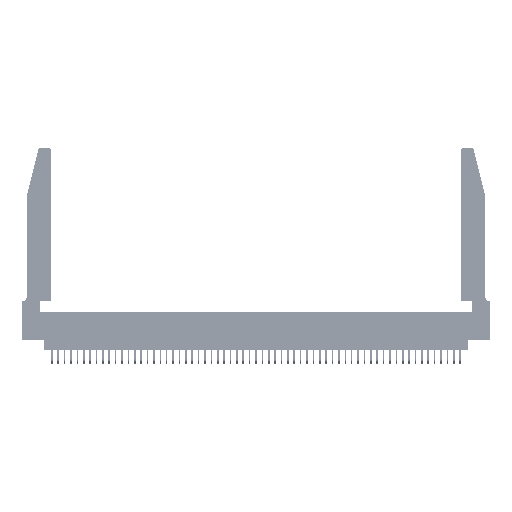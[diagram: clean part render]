
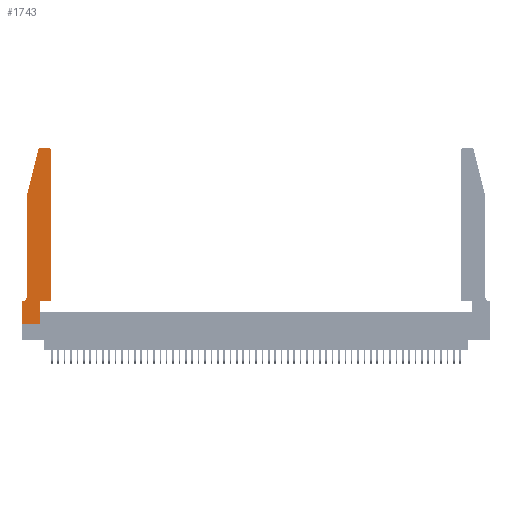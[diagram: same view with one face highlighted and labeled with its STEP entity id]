
A CAD part, top view. The second image highlights one B-rep face of the part: STEP entity #1743.
In plain terms, the highlighted planar face has unit normal (0, 0, 1).
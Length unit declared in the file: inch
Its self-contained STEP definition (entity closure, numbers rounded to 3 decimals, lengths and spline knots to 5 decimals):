
#750 = AXIS2_PLACEMENT_3D ( 'NONE', #9869, #39200, #14159 ) ;
#1013 = EDGE_CURVE ( 'NONE', #20179, #39010, #33569, .T. ) ;
#1075 = CARTESIAN_POINT ( 'NONE',  ( 0.2865, 0.35, 0.37 ) ) ;
#1083 = CIRCLE ( 'NONE', #750, 0.03 ) ;
#1559 = DIRECTION ( 'NONE',  ( 1., 0., 0. ) ) ;
#1733 = LINE ( 'NONE', #6909, #24325 ) ;
#1743 = ADVANCED_FACE ( 'NONE', ( #35420 ), #18550, .T. ) ;
#3032 = CARTESIAN_POINT ( 'NONE',  ( 0.2865, 0., 0.37 ) ) ;
#3134 = CARTESIAN_POINT ( 'NONE',  ( 0.0055, 0.42, 0.37 ) ) ;
#3614 = ORIENTED_EDGE ( 'NONE', *, *, #1013, .T. ) ;
#3737 = ORIENTED_EDGE ( 'NONE', *, *, #49846, .T. ) ;
#4103 = VECTOR ( 'NONE', #35746, 39.37008 ) ;
#4845 = EDGE_CURVE ( 'NONE', #18317, #18725, #52098, .T. ) ;
#5566 = CIRCLE ( 'NONE', #9182, 0.07 ) ;
#5987 = CARTESIAN_POINT ( 'NONE',  ( 0.0755, 2., 0.37 ) ) ;
#6481 = VECTOR ( 'NONE', #27525, 39.37008 ) ;
#6909 = CARTESIAN_POINT ( 'NONE',  ( 0.0755, 0.35, 0.37 ) ) ;
#7470 = DIRECTION ( 'NONE',  ( -1., 0., 0. ) ) ;
#7725 = ORIENTED_EDGE ( 'NONE', *, *, #34610, .T. ) ;
#7839 = LINE ( 'NONE', #23278, #6481 ) ;
#8473 = VECTOR ( 'NONE', #13533, 39.37008 ) ;
#8602 = CARTESIAN_POINT ( 'NONE',  ( 0.0755, 2., 0.37 ) ) ;
#9005 = CIRCLE ( 'NONE', #48217, 0.03 ) ;
#9182 = AXIS2_PLACEMENT_3D ( 'NONE', #3134, #32690, #7470 ) ;
#9738 = ORIENTED_EDGE ( 'NONE', *, *, #51817, .T. ) ;
#9869 = CARTESIAN_POINT ( 'NONE',  ( 0.4205, 2.72, 0.37 ) ) ;
#11455 = VERTEX_POINT ( 'NONE', #48692 ) ;
#11605 = VERTEX_POINT ( 'NONE', #8602 ) ;
#12984 = DIRECTION ( 'NONE',  ( -1., 0., 0. ) ) ;
#13178 = ORIENTED_EDGE ( 'NONE', *, *, #4845, .T. ) ;
#13533 = DIRECTION ( 'NONE',  ( 0., -1., 0. ) ) ;
#13627 = CARTESIAN_POINT ( 'NONE',  ( 0.4505, 2.72, 0.37 ) ) ;
#13728 = LINE ( 'NONE', #52797, #34656 ) ;
#14159 = DIRECTION ( 'NONE',  ( 1., 0., 0. ) ) ;
#14239 = DIRECTION ( 'NONE',  ( 0., 0., 1. ) ) ;
#14903 = VERTEX_POINT ( 'NONE', #26438 ) ;
#15467 = LINE ( 'NONE', #18952, #4103 ) ;
#15876 = LINE ( 'NONE', #5987, #45263 ) ;
#17391 = EDGE_CURVE ( 'NONE', #11605, #11455, #7839, .T. ) ;
#17397 = AXIS2_PLACEMENT_3D ( 'NONE', #47558, #26974, #1559 ) ;
#18262 = DIRECTION ( 'NONE',  ( 0., 1., 0. ) ) ;
#18317 = VERTEX_POINT ( 'NONE', #53519 ) ;
#18550 = PLANE ( 'NONE',  #17397 ) ;
#18725 = VERTEX_POINT ( 'NONE', #43685 ) ;
#18952 = CARTESIAN_POINT ( 'NONE',  ( 0.4505, 0.35, 0.37 ) ) ;
#19408 = CARTESIAN_POINT ( 'NONE',  ( 0., 0., 0.37 ) ) ;
#20179 = VERTEX_POINT ( 'NONE', #3032 ) ;
#20654 = ORIENTED_EDGE ( 'NONE', *, *, #25508, .T. ) ;
#20707 = VERTEX_POINT ( 'NONE', #53222 ) ;
#21090 = LINE ( 'NONE', #44475, #30902 ) ;
#22428 = EDGE_CURVE ( 'NONE', #14903, #11605, #15876, .T. ) ;
#22430 = VECTOR ( 'NONE', #18262, 39.37008 ) ;
#23278 = CARTESIAN_POINT ( 'NONE',  ( 0.0755, 2., 0.37 ) ) ;
#24325 = VECTOR ( 'NONE', #52880, 39.37008 ) ;
#25449 = ORIENTED_EDGE ( 'NONE', *, *, #30534, .T. ) ;
#25508 = EDGE_CURVE ( 'NONE', #36157, #47015, #15467, .T. ) ;
#26038 = ORIENTED_EDGE ( 'NONE', *, *, #45343, .T. ) ;
#26236 = VERTEX_POINT ( 'NONE', #19408 ) ;
#26438 = CARTESIAN_POINT ( 'NONE',  ( 0.25487, 2.72718, 0.37 ) ) ;
#26803 = VERTEX_POINT ( 'NONE', #30530 ) ;
#26974 = DIRECTION ( 'NONE',  ( 0., 0., 1. ) ) ;
#27525 = DIRECTION ( 'NONE',  ( 0., -1., 0. ) ) ;
#28639 = EDGE_CURVE ( 'NONE', #20707, #26236, #52987, .T. ) ;
#29494 = CARTESIAN_POINT ( 'NONE',  ( 0.2605, 2.75, 0.37 ) ) ;
#30530 = CARTESIAN_POINT ( 'NONE',  ( 0.0055, 0.35, 0.37 ) ) ;
#30534 = EDGE_CURVE ( 'NONE', #11455, #26803, #5566, .T. ) ;
#30902 = VECTOR ( 'NONE', #40261, 39.37008 ) ;
#32045 = DIRECTION ( 'NONE',  ( 1., 0., 0. ) ) ;
#32690 = DIRECTION ( 'NONE',  ( 0., 0., -1. ) ) ;
#33315 = ORIENTED_EDGE ( 'NONE', *, *, #28639, .T. ) ;
#33569 = LINE ( 'NONE', #1075, #22430 ) ;
#34374 = CARTESIAN_POINT ( 'NONE',  ( 0.4505, 0.35, 0.37 ) ) ;
#34610 = EDGE_CURVE ( 'NONE', #18725, #14903, #9005, .T. ) ;
#34656 = VECTOR ( 'NONE', #32045, 39.37008 ) ;
#35420 = FACE_OUTER_BOUND ( 'NONE', #43836, .T. ) ;
#35746 = DIRECTION ( 'NONE',  ( 0., 1., 0. ) ) ;
#36157 = VERTEX_POINT ( 'NONE', #34374 ) ;
#38428 = ORIENTED_EDGE ( 'NONE', *, *, #42991, .T. ) ;
#38730 = CARTESIAN_POINT ( 'NONE',  ( 0.2865, 0.35, 0.37 ) ) ;
#39010 = VERTEX_POINT ( 'NONE', #38730 ) ;
#39200 = DIRECTION ( 'NONE',  ( 0., 0., 1. ) ) ;
#39271 = CARTESIAN_POINT ( 'NONE',  ( 0.284, 2.72, 0.37 ) ) ;
#39619 = DIRECTION ( 'NONE',  ( -0.239, -0.971, 0. ) ) ;
#40261 = DIRECTION ( 'NONE',  ( 1., 0., 0. ) ) ;
#41028 = VECTOR ( 'NONE', #12984, 39.37008 ) ;
#42991 = EDGE_CURVE ( 'NONE', #26803, #20707, #1733, .T. ) ;
#43478 = DIRECTION ( 'NONE',  ( 1., 0., 0. ) ) ;
#43685 = CARTESIAN_POINT ( 'NONE',  ( 0.284, 2.75, 0.37 ) ) ;
#43836 = EDGE_LOOP ( 'NONE', ( #13178, #7725, #47736, #48548, #25449, #38428, #33315, #9738, #3614, #26038, #20654, #3737 ) ) ;
#44475 = CARTESIAN_POINT ( 'NONE',  ( 0.4505, 0.35, 0.37 ) ) ;
#45263 = VECTOR ( 'NONE', #39619, 39.37008 ) ;
#45343 = EDGE_CURVE ( 'NONE', #39010, #36157, #21090, .T. ) ;
#46954 = CARTESIAN_POINT ( 'NONE',  ( 0., 0., 0.37 ) ) ;
#47015 = VERTEX_POINT ( 'NONE', #13627 ) ;
#47558 = CARTESIAN_POINT ( 'NONE',  ( 0., 0.35, 0.37 ) ) ;
#47736 = ORIENTED_EDGE ( 'NONE', *, *, #22428, .T. ) ;
#48217 = AXIS2_PLACEMENT_3D ( 'NONE', #39271, #14239, #43478 ) ;
#48548 = ORIENTED_EDGE ( 'NONE', *, *, #17391, .T. ) ;
#48692 = CARTESIAN_POINT ( 'NONE',  ( 0.0755, 0.42, 0.37 ) ) ;
#49846 = EDGE_CURVE ( 'NONE', #47015, #18317, #1083, .T. ) ;
#51817 = EDGE_CURVE ( 'NONE', #26236, #20179, #13728, .T. ) ;
#52098 = LINE ( 'NONE', #29494, #41028 ) ;
#52797 = CARTESIAN_POINT ( 'NONE',  ( 0., 0., 0.37 ) ) ;
#52880 = DIRECTION ( 'NONE',  ( -1., 0., 0. ) ) ;
#52987 = LINE ( 'NONE', #46954, #8473 ) ;
#53222 = CARTESIAN_POINT ( 'NONE',  ( 0., 0.35, 0.37 ) ) ;
#53519 = CARTESIAN_POINT ( 'NONE',  ( 0.4205, 2.75, 0.37 ) ) ;
